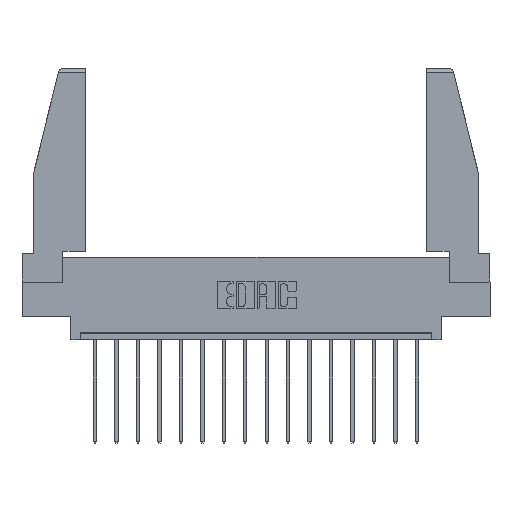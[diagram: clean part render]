
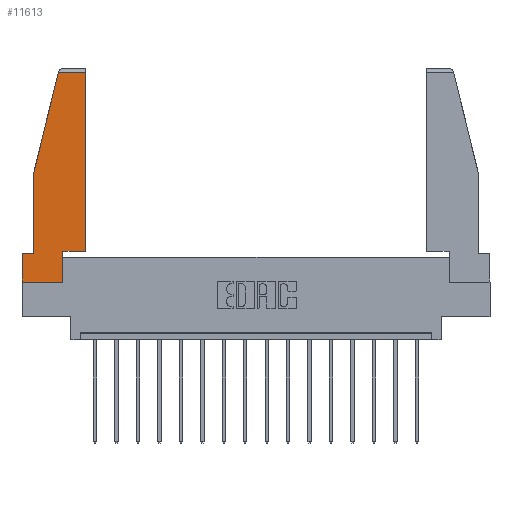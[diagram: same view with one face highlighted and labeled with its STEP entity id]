
A CAD part, top view. The second image highlights one B-rep face of the part: STEP entity #11613.
In plain terms, the highlighted planar face has unit normal (0, 0, 1).
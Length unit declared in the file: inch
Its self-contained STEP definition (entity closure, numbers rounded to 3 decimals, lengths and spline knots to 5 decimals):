
#16 = VERTEX_POINT ( 'NONE', #16578 ) ;
#100 = EDGE_CURVE ( 'NONE', #16, #2574, #11263, .T. ) ;
#461 = LINE ( 'NONE', #9534, #4809 ) ;
#682 = VECTOR ( 'NONE', #9349, 39.37008 ) ;
#851 = DIRECTION ( 'NONE',  ( 1., 0., 0. ) ) ;
#943 = LINE ( 'NONE', #15135, #7859 ) ;
#1379 = EDGE_CURVE ( 'NONE', #9345, #15217, #461, .T. ) ;
#1660 = ORIENTED_EDGE ( 'NONE', *, *, #12618, .T. ) ;
#1734 = LINE ( 'NONE', #7874, #8002 ) ;
#1846 = CARTESIAN_POINT ( 'NONE',  ( 0.461, 1.52, 0. ) ) ;
#1945 = ORIENTED_EDGE ( 'NONE', *, *, #100, .T. ) ;
#2281 = CARTESIAN_POINT ( 'NONE',  ( 0., 0.21, 0. ) ) ;
#2329 = LINE ( 'NONE', #2638, #10748 ) ;
#2574 = VERTEX_POINT ( 'NONE', #17761 ) ;
#2638 = CARTESIAN_POINT ( 'NONE',  ( 0., 0.21, 0. ) ) ;
#2928 = ORIENTED_EDGE ( 'NONE', *, *, #5867, .T. ) ;
#3775 = VECTOR ( 'NONE', #12703, 39.37008 ) ;
#3796 = ORIENTED_EDGE ( 'NONE', *, *, #17855, .T. ) ;
#4033 = AXIS2_PLACEMENT_3D ( 'NONE', #12330, #4122, #16499 ) ;
#4122 = DIRECTION ( 'NONE',  ( 0., 0., 1. ) ) ;
#4501 = VECTOR ( 'NONE', #7429, 39.37008 ) ;
#4559 = CARTESIAN_POINT ( 'NONE',  ( 0.086, 0.8, 0. ) ) ;
#4616 = CARTESIAN_POINT ( 'NONE',  ( 0., 0.21, 0. ) ) ;
#4765 = ORIENTED_EDGE ( 'NONE', *, *, #15935, .T. ) ;
#4809 = VECTOR ( 'NONE', #17764, 39.37008 ) ;
#5286 = DIRECTION ( 'NONE',  ( -1., 0., 0. ) ) ;
#5573 = VERTEX_POINT ( 'NONE', #2281 ) ;
#5593 = DIRECTION ( 'NONE',  ( 0., 1., 0. ) ) ;
#5867 = EDGE_CURVE ( 'NONE', #15104, #8514, #6993, .T. ) ;
#6266 = EDGE_LOOP ( 'NONE', ( #14099, #14501, #1660, #1945, #11838, #3796, #16109, #4765, #2928 ) ) ;
#6442 = DIRECTION ( 'NONE',  ( -0.239, -0.971, 0. ) ) ;
#6485 = EDGE_CURVE ( 'NONE', #8514, #9690, #15347, .T. ) ;
#6559 = CARTESIAN_POINT ( 'NONE',  ( 0., 0., 0. ) ) ;
#6638 = LINE ( 'NONE', #4616, #4501 ) ;
#6856 = CARTESIAN_POINT ( 'NONE',  ( 0.297, 0., 0. ) ) ;
#6993 = LINE ( 'NONE', #13372, #17082 ) ;
#7429 = DIRECTION ( 'NONE',  ( 0., -1., 0. ) ) ;
#7561 = LINE ( 'NONE', #17309, #10354 ) ;
#7653 = CARTESIAN_POINT ( 'NONE',  ( 0.461, 0.223, 0. ) ) ;
#7804 = CARTESIAN_POINT ( 'NONE',  ( 0.2636, 1.52, 0. ) ) ;
#7859 = VECTOR ( 'NONE', #5593, 39.37008 ) ;
#7874 = CARTESIAN_POINT ( 'NONE',  ( 0., 1.52, 0. ) ) ;
#8002 = VECTOR ( 'NONE', #5286, 39.37008 ) ;
#8034 = CARTESIAN_POINT ( 'NONE',  ( 0.461, 0.223, 0. ) ) ;
#8316 = VERTEX_POINT ( 'NONE', #7804 ) ;
#8514 = VERTEX_POINT ( 'NONE', #7653 ) ;
#9345 = VERTEX_POINT ( 'NONE', #6559 ) ;
#9349 = DIRECTION ( 'NONE',  ( 0., 1., 0. ) ) ;
#9487 = EDGE_CURVE ( 'NONE', #2574, #5573, #2329, .T. ) ;
#9534 = CARTESIAN_POINT ( 'NONE',  ( 0., 0., 0. ) ) ;
#9596 = PLANE ( 'NONE',  #4033 ) ;
#9690 = VERTEX_POINT ( 'NONE', #1846 ) ;
#10354 = VECTOR ( 'NONE', #6442, 39.37008 ) ;
#10748 = VECTOR ( 'NONE', #12186, 39.37008 ) ;
#11263 = LINE ( 'NONE', #4559, #3775 ) ;
#11613 = ADVANCED_FACE ( 'NONE', ( #14659 ), #9596, .T. ) ;
#11838 = ORIENTED_EDGE ( 'NONE', *, *, #9487, .T. ) ;
#12186 = DIRECTION ( 'NONE',  ( -1., 0., 0. ) ) ;
#12330 = CARTESIAN_POINT ( 'NONE',  ( 0., 0., 0. ) ) ;
#12618 = EDGE_CURVE ( 'NONE', #8316, #16, #7561, .T. ) ;
#12703 = DIRECTION ( 'NONE',  ( 0., -1., 0. ) ) ;
#12750 = EDGE_CURVE ( 'NONE', #9690, #8316, #1734, .T. ) ;
#13372 = CARTESIAN_POINT ( 'NONE',  ( 0.297, 0.223, 0. ) ) ;
#14099 = ORIENTED_EDGE ( 'NONE', *, *, #6485, .T. ) ;
#14501 = ORIENTED_EDGE ( 'NONE', *, *, #12750, .T. ) ;
#14659 = FACE_OUTER_BOUND ( 'NONE', #6266, .T. ) ;
#15104 = VERTEX_POINT ( 'NONE', #17305 ) ;
#15135 = CARTESIAN_POINT ( 'NONE',  ( 0.297, 0., 0. ) ) ;
#15217 = VERTEX_POINT ( 'NONE', #6856 ) ;
#15347 = LINE ( 'NONE', #8034, #682 ) ;
#15935 = EDGE_CURVE ( 'NONE', #15217, #15104, #943, .T. ) ;
#16109 = ORIENTED_EDGE ( 'NONE', *, *, #1379, .T. ) ;
#16499 = DIRECTION ( 'NONE',  ( 1., 0., 0. ) ) ;
#16578 = CARTESIAN_POINT ( 'NONE',  ( 0.086, 0.8, 0. ) ) ;
#17082 = VECTOR ( 'NONE', #851, 39.37008 ) ;
#17305 = CARTESIAN_POINT ( 'NONE',  ( 0.297, 0.223, 0. ) ) ;
#17309 = CARTESIAN_POINT ( 'NONE',  ( 0.271, 1.55, 0. ) ) ;
#17761 = CARTESIAN_POINT ( 'NONE',  ( 0.086, 0.21, 0. ) ) ;
#17764 = DIRECTION ( 'NONE',  ( 1., 0., 0. ) ) ;
#17855 = EDGE_CURVE ( 'NONE', #5573, #9345, #6638, .T. ) ;
